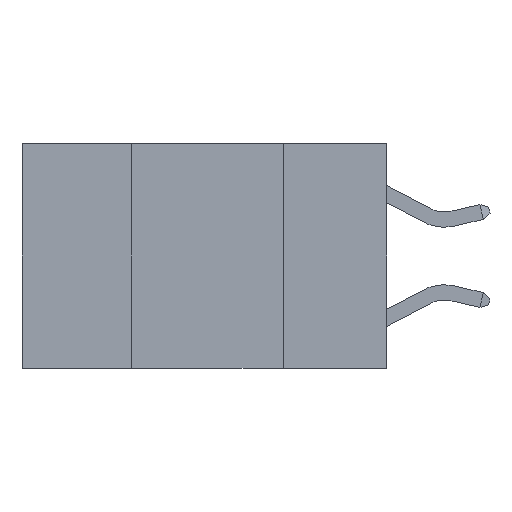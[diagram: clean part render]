
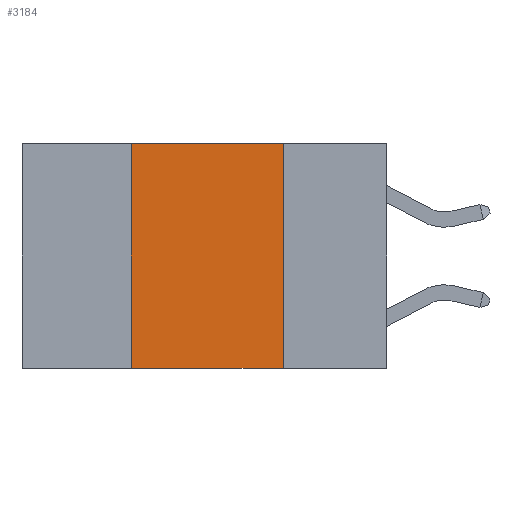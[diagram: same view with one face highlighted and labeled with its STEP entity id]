
A CAD part, left-side view. The second image highlights one B-rep face of the part: STEP entity #3184.
In plain terms, the highlighted planar face has unit normal (-1, 0, 0).
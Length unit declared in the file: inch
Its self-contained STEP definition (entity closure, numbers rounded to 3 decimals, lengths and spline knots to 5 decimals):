
#96 = DIRECTION ( 'NONE',  ( 0., -1., 0. ) ) ;
#138 = DIRECTION ( 'NONE',  ( 0., 0., 1. ) ) ;
#202 = CARTESIAN_POINT ( 'NONE',  ( 0., 0.17, -0.37 ) ) ;
#281 = EDGE_CURVE ( 'NONE', #7780, #3290, #1504, .T. ) ;
#321 = CARTESIAN_POINT ( 'NONE',  ( 0., 0.6, 0. ) ) ;
#425 = FACE_OUTER_BOUND ( 'NONE', #804, .T. ) ;
#501 = DIRECTION ( 'NONE',  ( 0., -1., 0. ) ) ;
#774 = LINE ( 'NONE', #2490, #8318 ) ;
#804 = EDGE_LOOP ( 'NONE', ( #2790, #8178, #2575, #2340 ) ) ;
#895 = LINE ( 'NONE', #3365, #8203 ) ;
#1366 = CARTESIAN_POINT ( 'NONE',  ( 0., 0.42, 0. ) ) ;
#1504 = LINE ( 'NONE', #1366, #4843 ) ;
#1752 = VERTEX_POINT ( 'NONE', #202 ) ;
#1795 = PLANE ( 'NONE',  #2500 ) ;
#2340 = ORIENTED_EDGE ( 'NONE', *, *, #8802, .T. ) ;
#2455 = VECTOR ( 'NONE', #96, 39.37008 ) ;
#2490 = CARTESIAN_POINT ( 'NONE',  ( 0., 0.17, 0. ) ) ;
#2500 = AXIS2_PLACEMENT_3D ( 'NONE', #321, #6775, #2530 ) ;
#2530 = DIRECTION ( 'NONE',  ( 0., 0., -1. ) ) ;
#2575 = ORIENTED_EDGE ( 'NONE', *, *, #281, .F. ) ;
#2790 = ORIENTED_EDGE ( 'NONE', *, *, #6798, .F. ) ;
#2889 = LINE ( 'NONE', #8580, #2455 ) ;
#3184 = ADVANCED_FACE ( 'NONE', ( #425 ), #1795, .F. ) ;
#3290 = VERTEX_POINT ( 'NONE', #6168 ) ;
#3365 = CARTESIAN_POINT ( 'NONE',  ( 0., 0.6, 0. ) ) ;
#3508 = CARTESIAN_POINT ( 'NONE',  ( 0., 0.42, -0.37 ) ) ;
#4533 = VERTEX_POINT ( 'NONE', #6028 ) ;
#4843 = VECTOR ( 'NONE', #138, 39.37008 ) ;
#6028 = CARTESIAN_POINT ( 'NONE',  ( 0., 0.17, 0. ) ) ;
#6168 = CARTESIAN_POINT ( 'NONE',  ( 0., 0.42, 0. ) ) ;
#6775 = DIRECTION ( 'NONE',  ( 1., 0., 0. ) ) ;
#6798 = EDGE_CURVE ( 'NONE', #4533, #1752, #774, .T. ) ;
#7060 = EDGE_CURVE ( 'NONE', #3290, #4533, #895, .T. ) ;
#7780 = VERTEX_POINT ( 'NONE', #3508 ) ;
#8117 = DIRECTION ( 'NONE',  ( 0., 0., -1. ) ) ;
#8178 = ORIENTED_EDGE ( 'NONE', *, *, #7060, .F. ) ;
#8203 = VECTOR ( 'NONE', #501, 39.37008 ) ;
#8318 = VECTOR ( 'NONE', #8117, 39.37008 ) ;
#8580 = CARTESIAN_POINT ( 'NONE',  ( 0., 0.6, -0.37 ) ) ;
#8802 = EDGE_CURVE ( 'NONE', #7780, #1752, #2889, .T. ) ;
